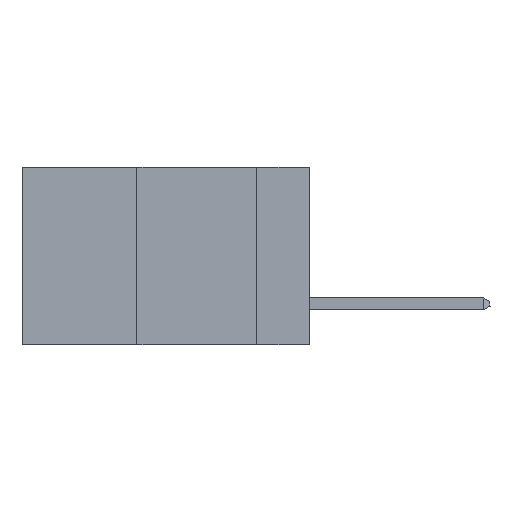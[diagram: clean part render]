
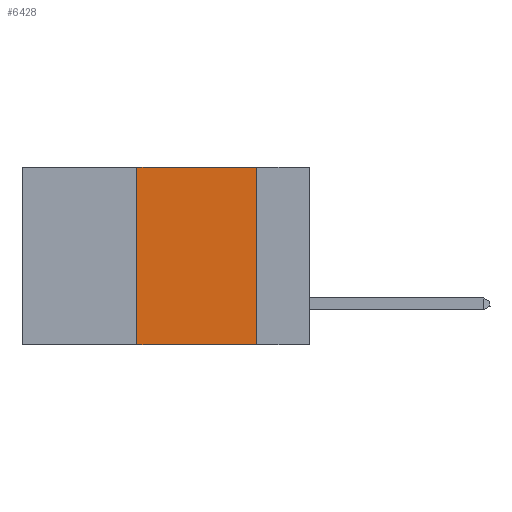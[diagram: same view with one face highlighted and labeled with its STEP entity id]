
A CAD part, left-side view. The second image highlights one B-rep face of the part: STEP entity #6428.
In plain terms, the highlighted planar face has unit normal (-1, 0, 0).
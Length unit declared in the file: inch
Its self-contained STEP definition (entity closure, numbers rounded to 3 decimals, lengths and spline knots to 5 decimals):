
#377 = VECTOR ( 'NONE', #1693, 39.37008 ) ;
#495 = EDGE_CURVE ( 'NONE', #25990, #21410, #18445, .T. ) ;
#1578 = LINE ( 'NONE', #15006, #8359 ) ;
#1660 = ORIENTED_EDGE ( 'NONE', *, *, #13980, .F. ) ;
#1693 = DIRECTION ( 'NONE',  ( 0., -1., 0. ) ) ;
#2087 = VERTEX_POINT ( 'NONE', #26295 ) ;
#2186 = CARTESIAN_POINT ( 'NONE',  ( 0., 0.11, 0. ) ) ;
#2557 = DIRECTION ( 'NONE',  ( 0., -1., 0. ) ) ;
#3630 = CARTESIAN_POINT ( 'NONE',  ( 0., 0.36, 0. ) ) ;
#5908 = CARTESIAN_POINT ( 'NONE',  ( 0., 0.11, 0. ) ) ;
#6428 = ADVANCED_FACE ( 'NONE', ( #21796 ), #20673, .F. ) ;
#6845 = VECTOR ( 'NONE', #2557, 39.37008 ) ;
#8359 = VECTOR ( 'NONE', #15807, 39.37008 ) ;
#9112 = ORIENTED_EDGE ( 'NONE', *, *, #12363, .T. ) ;
#9419 = ORIENTED_EDGE ( 'NONE', *, *, #25207, .F. ) ;
#10089 = DIRECTION ( 'NONE',  ( 0., 0., -1. ) ) ;
#11006 = CARTESIAN_POINT ( 'NONE',  ( 0., 0.11, -0.37 ) ) ;
#12288 = VECTOR ( 'NONE', #26686, 39.37008 ) ;
#12363 = EDGE_CURVE ( 'NONE', #2087, #21410, #17831, .T. ) ;
#13943 = LINE ( 'NONE', #18120, #377 ) ;
#13980 = EDGE_CURVE ( 'NONE', #2087, #24463, #1578, .T. ) ;
#14043 = DIRECTION ( 'NONE',  ( 1., 0., 0. ) ) ;
#15006 = CARTESIAN_POINT ( 'NONE',  ( 0., 0.36, 0. ) ) ;
#15807 = DIRECTION ( 'NONE',  ( 0., 0., 1. ) ) ;
#17831 = LINE ( 'NONE', #24178, #6845 ) ;
#18120 = CARTESIAN_POINT ( 'NONE',  ( 0., 0.6, 0. ) ) ;
#18445 = LINE ( 'NONE', #5908, #12288 ) ;
#20673 = PLANE ( 'NONE',  #21926 ) ;
#20856 = ORIENTED_EDGE ( 'NONE', *, *, #495, .F. ) ;
#21410 = VERTEX_POINT ( 'NONE', #11006 ) ;
#21796 = FACE_OUTER_BOUND ( 'NONE', #24412, .T. ) ;
#21926 = AXIS2_PLACEMENT_3D ( 'NONE', #22717, #14043, #10089 ) ;
#22717 = CARTESIAN_POINT ( 'NONE',  ( 0., 0.6, 0. ) ) ;
#24178 = CARTESIAN_POINT ( 'NONE',  ( 0., 0.6, -0.37 ) ) ;
#24412 = EDGE_LOOP ( 'NONE', ( #20856, #9419, #1660, #9112 ) ) ;
#24463 = VERTEX_POINT ( 'NONE', #3630 ) ;
#25207 = EDGE_CURVE ( 'NONE', #24463, #25990, #13943, .T. ) ;
#25990 = VERTEX_POINT ( 'NONE', #2186 ) ;
#26295 = CARTESIAN_POINT ( 'NONE',  ( 0., 0.36, -0.37 ) ) ;
#26686 = DIRECTION ( 'NONE',  ( 0., 0., -1. ) ) ;
